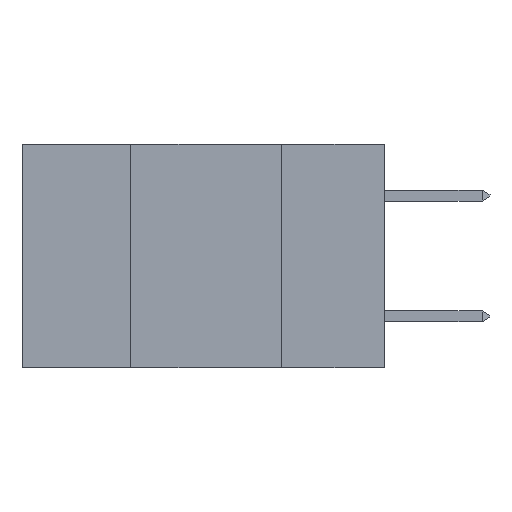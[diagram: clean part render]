
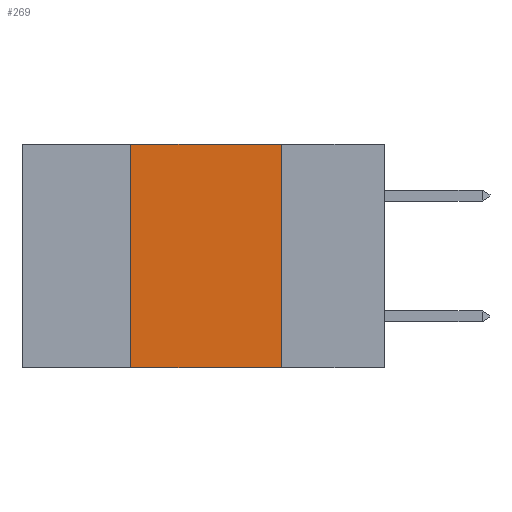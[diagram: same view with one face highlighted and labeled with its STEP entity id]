
A CAD part, left-side view. The second image highlights one B-rep face of the part: STEP entity #269.
In plain terms, the highlighted planar face has unit normal (-1, 0, 0).
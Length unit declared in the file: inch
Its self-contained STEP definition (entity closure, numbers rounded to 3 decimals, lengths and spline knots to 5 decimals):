
#108 = EDGE_LOOP ( 'NONE', ( #4597, #9562, #5740, #4098 ) ) ;
#109 = CARTESIAN_POINT ( 'NONE',  ( 0., 0.6, 0. ) ) ;
#269 = ADVANCED_FACE ( 'NONE', ( #5152 ), #843, .F. ) ;
#533 = LINE ( 'NONE', #1826, #877 ) ;
#843 = PLANE ( 'NONE',  #6241 ) ;
#877 = VECTOR ( 'NONE', #1800, 39.37008 ) ;
#1800 = DIRECTION ( 'NONE',  ( 0., 0., -1. ) ) ;
#1826 = CARTESIAN_POINT ( 'NONE',  ( 0., 0.17, 0. ) ) ;
#1880 = LINE ( 'NONE', #9029, #9688 ) ;
#2267 = CARTESIAN_POINT ( 'NONE',  ( 0., 0.17, -0.37 ) ) ;
#3191 = VERTEX_POINT ( 'NONE', #9807 ) ;
#4098 = ORIENTED_EDGE ( 'NONE', *, *, #9611, .T. ) ;
#4290 = EDGE_CURVE ( 'NONE', #3191, #10992, #5698, .T. ) ;
#4493 = DIRECTION ( 'NONE',  ( 0., -1., 0. ) ) ;
#4597 = ORIENTED_EDGE ( 'NONE', *, *, #6460, .F. ) ;
#4945 = DIRECTION ( 'NONE',  ( 1., 0., 0. ) ) ;
#5049 = VERTEX_POINT ( 'NONE', #2267 ) ;
#5152 = FACE_OUTER_BOUND ( 'NONE', #108, .T. ) ;
#5616 = VERTEX_POINT ( 'NONE', #8440 ) ;
#5698 = LINE ( 'NONE', #5758, #9879 ) ;
#5714 = DIRECTION ( 'NONE',  ( 0., 0., 1. ) ) ;
#5738 = DIRECTION ( 'NONE',  ( 0., 0., -1. ) ) ;
#5740 = ORIENTED_EDGE ( 'NONE', *, *, #4290, .F. ) ;
#5758 = CARTESIAN_POINT ( 'NONE',  ( 0., 0.42, 0. ) ) ;
#6241 = AXIS2_PLACEMENT_3D ( 'NONE', #109, #4945, #5738 ) ;
#6460 = EDGE_CURVE ( 'NONE', #5616, #5049, #533, .T. ) ;
#7486 = VECTOR ( 'NONE', #4493, 39.37008 ) ;
#7683 = CARTESIAN_POINT ( 'NONE',  ( 0., 0.6, 0. ) ) ;
#8440 = CARTESIAN_POINT ( 'NONE',  ( 0., 0.17, 0. ) ) ;
#8791 = CARTESIAN_POINT ( 'NONE',  ( 0., 0.42, 0. ) ) ;
#9029 = CARTESIAN_POINT ( 'NONE',  ( 0., 0.6, -0.37 ) ) ;
#9562 = ORIENTED_EDGE ( 'NONE', *, *, #9855, .F. ) ;
#9571 = LINE ( 'NONE', #7683, #7486 ) ;
#9611 = EDGE_CURVE ( 'NONE', #3191, #5049, #1880, .T. ) ;
#9688 = VECTOR ( 'NONE', #9794, 39.37008 ) ;
#9794 = DIRECTION ( 'NONE',  ( 0., -1., 0. ) ) ;
#9807 = CARTESIAN_POINT ( 'NONE',  ( 0., 0.42, -0.37 ) ) ;
#9855 = EDGE_CURVE ( 'NONE', #10992, #5616, #9571, .T. ) ;
#9879 = VECTOR ( 'NONE', #5714, 39.37008 ) ;
#10992 = VERTEX_POINT ( 'NONE', #8791 ) ;
